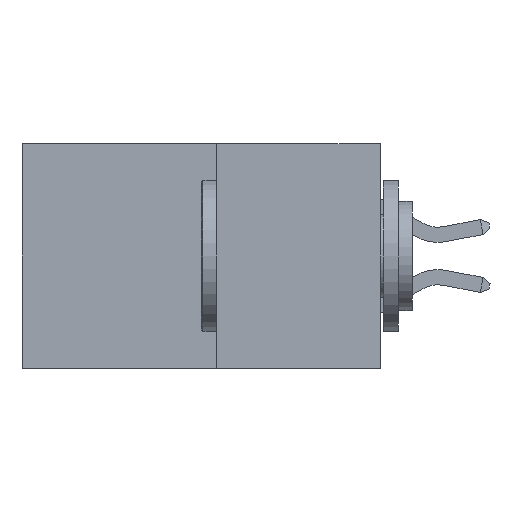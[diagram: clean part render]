
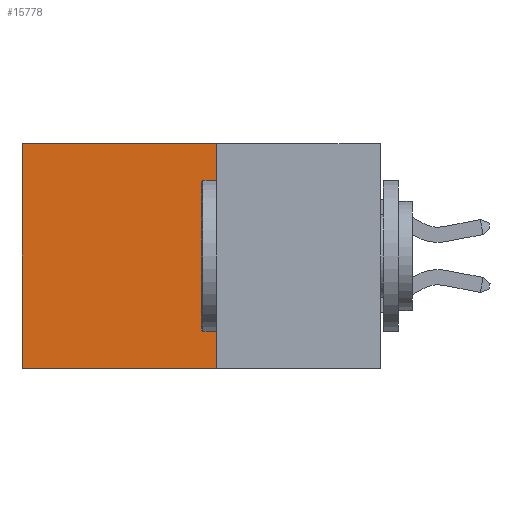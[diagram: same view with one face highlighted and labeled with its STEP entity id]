
A CAD part, left-side view. The second image highlights one B-rep face of the part: STEP entity #15778.
In plain terms, the highlighted planar face has unit normal (-1, 0, 0).
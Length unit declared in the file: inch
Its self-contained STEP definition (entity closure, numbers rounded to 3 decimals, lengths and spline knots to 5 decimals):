
#81 = ORIENTED_EDGE ( 'NONE', *, *, #17661, .F. ) ;
#216 = FACE_OUTER_BOUND ( 'NONE', #10114, .T. ) ;
#667 = ORIENTED_EDGE ( 'NONE', *, *, #10028, .T. ) ;
#803 = VERTEX_POINT ( 'NONE', #3912 ) ;
#2487 = LINE ( 'NONE', #6317, #17171 ) ;
#2499 = LINE ( 'NONE', #11425, #9719 ) ;
#2835 = DIRECTION ( 'NONE',  ( 0., 1., 0. ) ) ;
#3912 = CARTESIAN_POINT ( 'NONE',  ( 0.277, 0.59, -0.37 ) ) ;
#5040 = VERTEX_POINT ( 'NONE', #6113 ) ;
#5145 = VECTOR ( 'NONE', #12737, 39.37008 ) ;
#5753 = EDGE_CURVE ( 'NONE', #8729, #8276, #16446, .T. ) ;
#6113 = CARTESIAN_POINT ( 'NONE',  ( 0.277, 0.27, -0.37 ) ) ;
#6317 = CARTESIAN_POINT ( 'NONE',  ( 0.277, 0.59, -0.37 ) ) ;
#6873 = DIRECTION ( 'NONE',  ( 0., 0., -1. ) ) ;
#7834 = CARTESIAN_POINT ( 'NONE',  ( 0.277, 0.27, 0. ) ) ;
#7935 = LINE ( 'NONE', #16514, #11240 ) ;
#8276 = VERTEX_POINT ( 'NONE', #11054 ) ;
#8608 = DIRECTION ( 'NONE',  ( 0., 0., -1. ) ) ;
#8657 = EDGE_CURVE ( 'NONE', #5040, #803, #7935, .T. ) ;
#8729 = VERTEX_POINT ( 'NONE', #11354 ) ;
#9719 = VECTOR ( 'NONE', #8608, 39.37008 ) ;
#10028 = EDGE_CURVE ( 'NONE', #8276, #803, #2487, .T. ) ;
#10114 = EDGE_LOOP ( 'NONE', ( #667, #17239, #81, #12677 ) ) ;
#11054 = CARTESIAN_POINT ( 'NONE',  ( 0.277, 0.59, 0. ) ) ;
#11240 = VECTOR ( 'NONE', #2835, 39.37008 ) ;
#11354 = CARTESIAN_POINT ( 'NONE',  ( 0.277, 0.27, 0. ) ) ;
#11425 = CARTESIAN_POINT ( 'NONE',  ( 0.277, 0.27, -0.37 ) ) ;
#12677 = ORIENTED_EDGE ( 'NONE', *, *, #5753, .T. ) ;
#12737 = DIRECTION ( 'NONE',  ( 0., 1., 0. ) ) ;
#13749 = DIRECTION ( 'NONE',  ( 0., 0., -1. ) ) ;
#13774 = DIRECTION ( 'NONE',  ( 1., 0., 0. ) ) ;
#13961 = CARTESIAN_POINT ( 'NONE',  ( 0.277, 0.27, -0.37 ) ) ;
#15285 = PLANE ( 'NONE',  #16301 ) ;
#15778 = ADVANCED_FACE ( 'NONE', ( #216 ), #15285, .F. ) ;
#16301 = AXIS2_PLACEMENT_3D ( 'NONE', #13961, #13774, #13749 ) ;
#16446 = LINE ( 'NONE', #7834, #5145 ) ;
#16514 = CARTESIAN_POINT ( 'NONE',  ( 0.277, 0.27, -0.37 ) ) ;
#17171 = VECTOR ( 'NONE', #6873, 39.37008 ) ;
#17239 = ORIENTED_EDGE ( 'NONE', *, *, #8657, .F. ) ;
#17661 = EDGE_CURVE ( 'NONE', #8729, #5040, #2499, .T. ) ;
